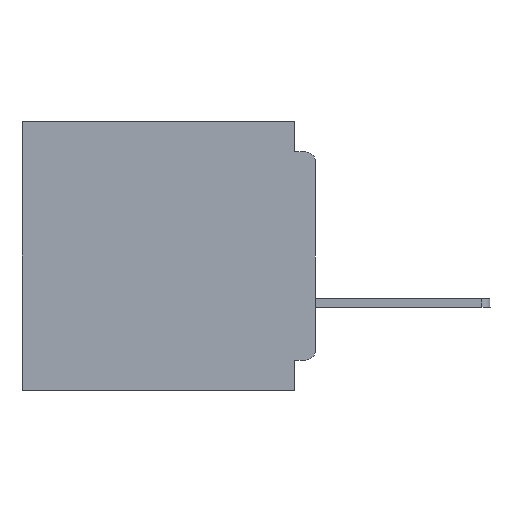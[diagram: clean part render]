
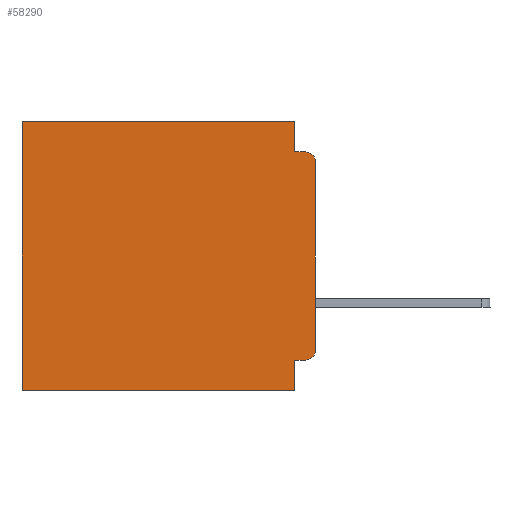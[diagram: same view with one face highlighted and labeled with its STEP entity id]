
A CAD part, left-side view. The second image highlights one B-rep face of the part: STEP entity #58290.
In plain terms, the highlighted planar face has unit normal (-1, 0, 0).
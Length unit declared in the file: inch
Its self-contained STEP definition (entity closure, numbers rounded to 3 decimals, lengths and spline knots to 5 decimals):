
#1004 = AXIS2_PLACEMENT_3D ( 'NONE', #58198, #27894, #63207 ) ;
#1154 = DIRECTION ( 'NONE',  ( 1., 0., 0. ) ) ;
#1844 = DIRECTION ( 'NONE',  ( 0., 0., -1. ) ) ;
#1970 = VERTEX_POINT ( 'NONE', #26200 ) ;
#2144 = CARTESIAN_POINT ( 'NONE',  ( 0.3, 0.015, -0.06 ) ) ;
#3605 = ORIENTED_EDGE ( 'NONE', *, *, #64323, .T. ) ;
#3667 = ORIENTED_EDGE ( 'NONE', *, *, #38274, .F. ) ;
#3932 = LINE ( 'NONE', #43038, #29538 ) ;
#4939 = VERTEX_POINT ( 'NONE', #65167 ) ;
#5322 = LINE ( 'NONE', #58757, #44391 ) ;
#6340 = CARTESIAN_POINT ( 'NONE',  ( 0.3, 0.437, 0. ) ) ;
#6572 = DIRECTION ( 'NONE',  ( 0., 1., 0. ) ) ;
#6831 = CARTESIAN_POINT ( 'NONE',  ( 0.3, 0.031, -0.4 ) ) ;
#7352 = DIRECTION ( 'NONE',  ( 0., 0., -1. ) ) ;
#9171 = ORIENTED_EDGE ( 'NONE', *, *, #53103, .F. ) ;
#9244 = EDGE_CURVE ( 'NONE', #15582, #21251, #3932, .T. ) ;
#9310 = VERTEX_POINT ( 'NONE', #43466 ) ;
#9327 = AXIS2_PLACEMENT_3D ( 'NONE', #2144, #37893, #7352 ) ;
#10224 = CARTESIAN_POINT ( 'NONE',  ( 0.3, 0.031, 0. ) ) ;
#10850 = CARTESIAN_POINT ( 'NONE',  ( 0.3, 0.031, 0. ) ) ;
#11277 = PLANE ( 'NONE',  #55423 ) ;
#13430 = CIRCLE ( 'NONE', #9327, 0.015 ) ;
#14559 = FACE_OUTER_BOUND ( 'NONE', #50431, .T. ) ;
#15582 = VERTEX_POINT ( 'NONE', #43647 ) ;
#15899 = LINE ( 'NONE', #46883, #29477 ) ;
#16253 = CARTESIAN_POINT ( 'NONE',  ( 0.3, 0., -0.06 ) ) ;
#17284 = DIRECTION ( 'NONE',  ( 0., -1., 0. ) ) ;
#18363 = VERTEX_POINT ( 'NONE', #19204 ) ;
#18858 = VECTOR ( 'NONE', #43542, 39.37008 ) ;
#19204 = CARTESIAN_POINT ( 'NONE',  ( 0.3, 0.031, -0.355 ) ) ;
#20818 = VECTOR ( 'NONE', #1844, 39.37008 ) ;
#21251 = VERTEX_POINT ( 'NONE', #36712 ) ;
#21712 = VECTOR ( 'NONE', #46494, 39.37008 ) ;
#22454 = LINE ( 'NONE', #6831, #20818 ) ;
#23308 = CARTESIAN_POINT ( 'NONE',  ( 0.3, 0., -0.4 ) ) ;
#24662 = VECTOR ( 'NONE', #62812, 39.37008 ) ;
#26200 = CARTESIAN_POINT ( 'NONE',  ( 0.3, 0.015, -0.045 ) ) ;
#27488 = CARTESIAN_POINT ( 'NONE',  ( 0.3, 0., -0.355 ) ) ;
#27542 = CARTESIAN_POINT ( 'NONE',  ( 0.3, 0.031, -0.045 ) ) ;
#27894 = DIRECTION ( 'NONE',  ( -1., 0., 0. ) ) ;
#28441 = DIRECTION ( 'NONE',  ( 0., 0., -1. ) ) ;
#28818 = EDGE_CURVE ( 'NONE', #9310, #18363, #36619, .T. ) ;
#29477 = VECTOR ( 'NONE', #17284, 39.37008 ) ;
#29538 = VECTOR ( 'NONE', #48112, 39.37008 ) ;
#30102 = VERTEX_POINT ( 'NONE', #27542 ) ;
#30278 = CIRCLE ( 'NONE', #1004, 0.015 ) ;
#31831 = CARTESIAN_POINT ( 'NONE',  ( 0.3, 0., -0.4 ) ) ;
#32887 = VERTEX_POINT ( 'NONE', #6340 ) ;
#33073 = ORIENTED_EDGE ( 'NONE', *, *, #9244, .F. ) ;
#34762 = EDGE_CURVE ( 'NONE', #54788, #1970, #13430, .T. ) ;
#35523 = ORIENTED_EDGE ( 'NONE', *, *, #34762, .T. ) ;
#35658 = LINE ( 'NONE', #23308, #18858 ) ;
#36619 = LINE ( 'NONE', #27488, #24662 ) ;
#36712 = CARTESIAN_POINT ( 'NONE',  ( 0.3, 0.437, -0.4 ) ) ;
#36930 = DIRECTION ( 'NONE',  ( 0., 0., -1. ) ) ;
#37893 = DIRECTION ( 'NONE',  ( -1., 0., 0. ) ) ;
#38274 = EDGE_CURVE ( 'NONE', #48753, #30102, #60551, .T. ) ;
#39892 = EDGE_CURVE ( 'NONE', #30102, #1970, #15899, .T. ) ;
#41230 = ORIENTED_EDGE ( 'NONE', *, *, #50979, .T. ) ;
#43038 = CARTESIAN_POINT ( 'NONE',  ( 0.3, 0., -0.4 ) ) ;
#43466 = CARTESIAN_POINT ( 'NONE',  ( 0.3, 0.015, -0.355 ) ) ;
#43542 = DIRECTION ( 'NONE',  ( 0., 0., -1. ) ) ;
#43647 = CARTESIAN_POINT ( 'NONE',  ( 0.3, 0.031, -0.4 ) ) ;
#43794 = ORIENTED_EDGE ( 'NONE', *, *, #28818, .F. ) ;
#43906 = VECTOR ( 'NONE', #6572, 39.37008 ) ;
#44391 = VECTOR ( 'NONE', #28441, 39.37008 ) ;
#44705 = EDGE_CURVE ( 'NONE', #48753, #32887, #58893, .T. ) ;
#45644 = ORIENTED_EDGE ( 'NONE', *, *, #44705, .T. ) ;
#46494 = DIRECTION ( 'NONE',  ( 0., 0., -1. ) ) ;
#46883 = CARTESIAN_POINT ( 'NONE',  ( 0.3, 0., -0.045 ) ) ;
#48112 = DIRECTION ( 'NONE',  ( 0., 1., 0. ) ) ;
#48753 = VERTEX_POINT ( 'NONE', #10224 ) ;
#50431 = EDGE_LOOP ( 'NONE', ( #65924, #35523, #50445, #3667, #45644, #41230, #33073, #9171, #43794, #3605 ) ) ;
#50445 = ORIENTED_EDGE ( 'NONE', *, *, #39892, .F. ) ;
#50969 = EDGE_CURVE ( 'NONE', #54788, #4939, #35658, .T. ) ;
#50979 = EDGE_CURVE ( 'NONE', #32887, #21251, #5322, .T. ) ;
#53103 = EDGE_CURVE ( 'NONE', #18363, #15582, #22454, .T. ) ;
#54788 = VERTEX_POINT ( 'NONE', #16253 ) ;
#55423 = AXIS2_PLACEMENT_3D ( 'NONE', #31831, #1154, #36930 ) ;
#58198 = CARTESIAN_POINT ( 'NONE',  ( 0.3, 0.015, -0.34 ) ) ;
#58290 = ADVANCED_FACE ( 'NONE', ( #14559 ), #11277, .F. ) ;
#58757 = CARTESIAN_POINT ( 'NONE',  ( 0.3, 0.437, -0.4 ) ) ;
#58893 = LINE ( 'NONE', #62267, #43906 ) ;
#60551 = LINE ( 'NONE', #10850, #21712 ) ;
#62267 = CARTESIAN_POINT ( 'NONE',  ( 0.3, 0., 0. ) ) ;
#62812 = DIRECTION ( 'NONE',  ( 0., 1., 0. ) ) ;
#63207 = DIRECTION ( 'NONE',  ( 0., 0., -1. ) ) ;
#64323 = EDGE_CURVE ( 'NONE', #9310, #4939, #30278, .T. ) ;
#65167 = CARTESIAN_POINT ( 'NONE',  ( 0.3, 0., -0.34 ) ) ;
#65924 = ORIENTED_EDGE ( 'NONE', *, *, #50969, .F. ) ;
